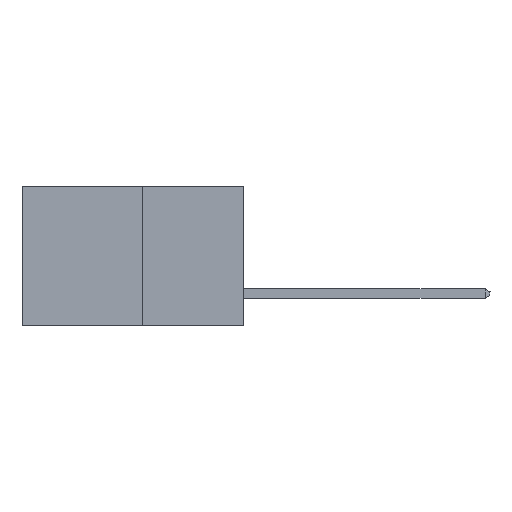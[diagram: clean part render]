
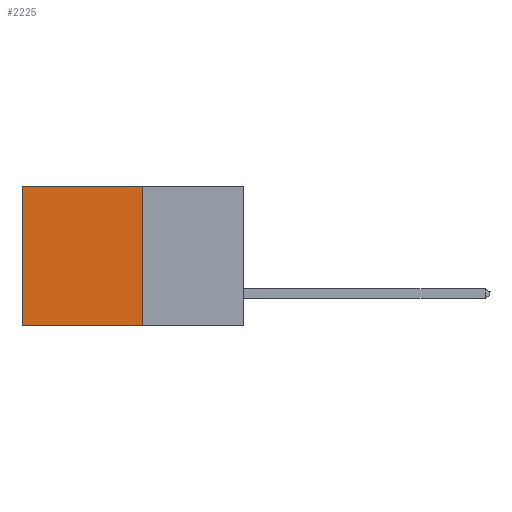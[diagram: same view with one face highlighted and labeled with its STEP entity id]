
A CAD part, left-side view. The second image highlights one B-rep face of the part: STEP entity #2225.
In plain terms, the highlighted planar face has unit normal (-1, 0, 0).
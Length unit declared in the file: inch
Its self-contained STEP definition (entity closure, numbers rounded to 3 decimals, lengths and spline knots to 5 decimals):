
#62 = DIRECTION ( 'NONE',  ( 1., 0., 0. ) ) ;
#188 = PLANE ( 'NONE',  #537 ) ;
#537 = AXIS2_PLACEMENT_3D ( 'NONE', #6463, #62, #11239 ) ;
#741 = EDGE_CURVE ( 'NONE', #1275, #14268, #2697, .T. ) ;
#1275 = VERTEX_POINT ( 'NONE', #9137 ) ;
#2225 = ADVANCED_FACE ( 'NONE', ( #4166 ), #188, .F. ) ;
#2489 = EDGE_CURVE ( 'NONE', #5846, #1275, #3971, .T. ) ;
#2697 = LINE ( 'NONE', #12637, #8495 ) ;
#2755 = CARTESIAN_POINT ( 'NONE',  ( 0.277, 0.27, 0. ) ) ;
#3695 = ORIENTED_EDGE ( 'NONE', *, *, #2489, .F. ) ;
#3971 = LINE ( 'NONE', #10899, #6754 ) ;
#4166 = FACE_OUTER_BOUND ( 'NONE', #11743, .T. ) ;
#4712 = DIRECTION ( 'NONE',  ( 0., 1., 0. ) ) ;
#5583 = VERTEX_POINT ( 'NONE', #13630 ) ;
#5846 = VERTEX_POINT ( 'NONE', #2755 ) ;
#6463 = CARTESIAN_POINT ( 'NONE',  ( 0.277, 0.27, -0.37 ) ) ;
#6481 = ORIENTED_EDGE ( 'NONE', *, *, #14319, .T. ) ;
#6625 = DIRECTION ( 'NONE',  ( 0., 1., 0. ) ) ;
#6754 = VECTOR ( 'NONE', #14058, 39.37008 ) ;
#6854 = ORIENTED_EDGE ( 'NONE', *, *, #12871, .T. ) ;
#8412 = VECTOR ( 'NONE', #12559, 39.37008 ) ;
#8495 = VECTOR ( 'NONE', #4712, 39.37008 ) ;
#9137 = CARTESIAN_POINT ( 'NONE',  ( 0.277, 0.27, -0.37 ) ) ;
#9372 = ORIENTED_EDGE ( 'NONE', *, *, #741, .F. ) ;
#10262 = CARTESIAN_POINT ( 'NONE',  ( 0.277, 0.59, -0.37 ) ) ;
#10899 = CARTESIAN_POINT ( 'NONE',  ( 0.277, 0.27, -0.37 ) ) ;
#11239 = DIRECTION ( 'NONE',  ( 0., 0., -1. ) ) ;
#11442 = CARTESIAN_POINT ( 'NONE',  ( 0.277, 0.59, -0.37 ) ) ;
#11743 = EDGE_LOOP ( 'NONE', ( #6481, #9372, #3695, #6854 ) ) ;
#12037 = LINE ( 'NONE', #11442, #8412 ) ;
#12559 = DIRECTION ( 'NONE',  ( 0., 0., -1. ) ) ;
#12637 = CARTESIAN_POINT ( 'NONE',  ( 0.277, 0.27, -0.37 ) ) ;
#12871 = EDGE_CURVE ( 'NONE', #5846, #5583, #13254, .T. ) ;
#13214 = CARTESIAN_POINT ( 'NONE',  ( 0.277, 0.27, 0. ) ) ;
#13254 = LINE ( 'NONE', #13214, #13958 ) ;
#13630 = CARTESIAN_POINT ( 'NONE',  ( 0.277, 0.59, 0. ) ) ;
#13958 = VECTOR ( 'NONE', #6625, 39.37008 ) ;
#14058 = DIRECTION ( 'NONE',  ( 0., 0., -1. ) ) ;
#14268 = VERTEX_POINT ( 'NONE', #10262 ) ;
#14319 = EDGE_CURVE ( 'NONE', #5583, #14268, #12037, .T. ) ;
